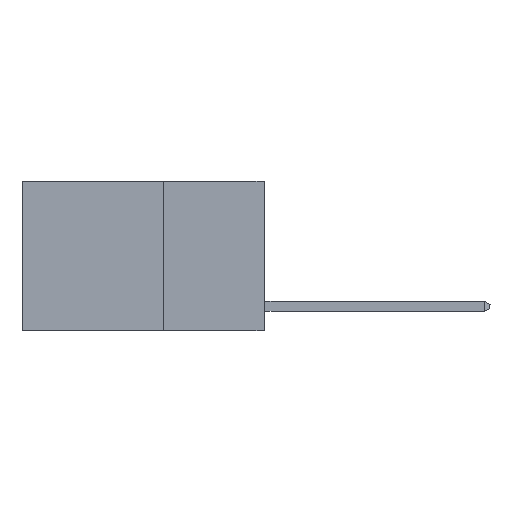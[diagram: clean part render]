
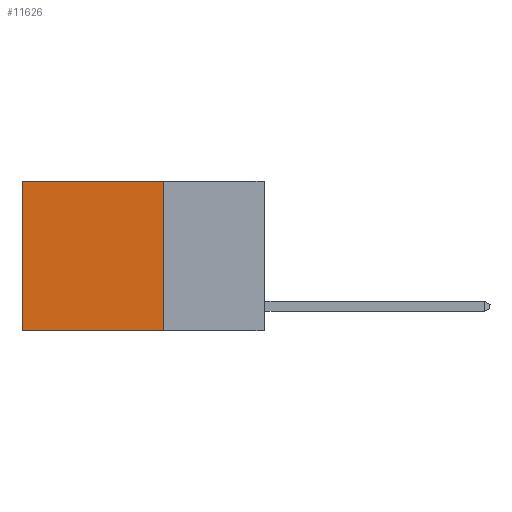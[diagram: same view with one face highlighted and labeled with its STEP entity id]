
A CAD part, left-side view. The second image highlights one B-rep face of the part: STEP entity #11626.
In plain terms, the highlighted planar face has unit normal (-1, 0, 0).
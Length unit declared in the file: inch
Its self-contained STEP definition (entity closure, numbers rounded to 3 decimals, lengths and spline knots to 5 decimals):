
#86 = VECTOR ( 'NONE', #15028, 39.37008 ) ;
#139 = CARTESIAN_POINT ( 'NONE',  ( 0.2625, 0.25, 0. ) ) ;
#588 = ORIENTED_EDGE ( 'NONE', *, *, #14624, .T. ) ;
#840 = CARTESIAN_POINT ( 'NONE',  ( 0.2625, 0.25, 0. ) ) ;
#1755 = CARTESIAN_POINT ( 'NONE',  ( 0.2625, 0.6, 0. ) ) ;
#2412 = CARTESIAN_POINT ( 'NONE',  ( 0.2625, 0.25, -0.37 ) ) ;
#3845 = EDGE_CURVE ( 'NONE', #11852, #13822, #16744, .T. ) ;
#4538 = DIRECTION ( 'NONE',  ( 0., 1., 0. ) ) ;
#4725 = ORIENTED_EDGE ( 'NONE', *, *, #19110, .T. ) ;
#5920 = CARTESIAN_POINT ( 'NONE',  ( 0.2625, 0.25, -0.37 ) ) ;
#6238 = DIRECTION ( 'NONE',  ( 1., 0., 0. ) ) ;
#6312 = CARTESIAN_POINT ( 'NONE',  ( 0.2625, 0.25, 0. ) ) ;
#6634 = ORIENTED_EDGE ( 'NONE', *, *, #25311, .F. ) ;
#7064 = VECTOR ( 'NONE', #17626, 39.37008 ) ;
#7552 = PLANE ( 'NONE',  #11158 ) ;
#9342 = LINE ( 'NONE', #139, #12175 ) ;
#9843 = VECTOR ( 'NONE', #4538, 39.37008 ) ;
#10043 = DIRECTION ( 'NONE',  ( 0., 1., 0. ) ) ;
#11158 = AXIS2_PLACEMENT_3D ( 'NONE', #6312, #6238, #12051 ) ;
#11354 = VERTEX_POINT ( 'NONE', #1755 ) ;
#11455 = LINE ( 'NONE', #840, #86 ) ;
#11626 = ADVANCED_FACE ( 'NONE', ( #12758 ), #7552, .F. ) ;
#11852 = VERTEX_POINT ( 'NONE', #5920 ) ;
#12051 = DIRECTION ( 'NONE',  ( 0., 0., -1. ) ) ;
#12175 = VECTOR ( 'NONE', #10043, 39.37008 ) ;
#12758 = FACE_OUTER_BOUND ( 'NONE', #18139, .T. ) ;
#13822 = VERTEX_POINT ( 'NONE', #16619 ) ;
#14624 = EDGE_CURVE ( 'NONE', #25299, #11354, #9342, .T. ) ;
#15028 = DIRECTION ( 'NONE',  ( 0., 0., -1. ) ) ;
#16203 = LINE ( 'NONE', #23484, #7064 ) ;
#16619 = CARTESIAN_POINT ( 'NONE',  ( 0.2625, 0.6, -0.37 ) ) ;
#16744 = LINE ( 'NONE', #2412, #9843 ) ;
#17626 = DIRECTION ( 'NONE',  ( 0., 0., -1. ) ) ;
#18139 = EDGE_LOOP ( 'NONE', ( #4725, #19864, #6634, #588 ) ) ;
#19110 = EDGE_CURVE ( 'NONE', #11354, #13822, #16203, .T. ) ;
#19864 = ORIENTED_EDGE ( 'NONE', *, *, #3845, .F. ) ;
#22830 = CARTESIAN_POINT ( 'NONE',  ( 0.2625, 0.25, 0. ) ) ;
#23484 = CARTESIAN_POINT ( 'NONE',  ( 0.2625, 0.6, 0. ) ) ;
#25299 = VERTEX_POINT ( 'NONE', #22830 ) ;
#25311 = EDGE_CURVE ( 'NONE', #25299, #11852, #11455, .T. ) ;
